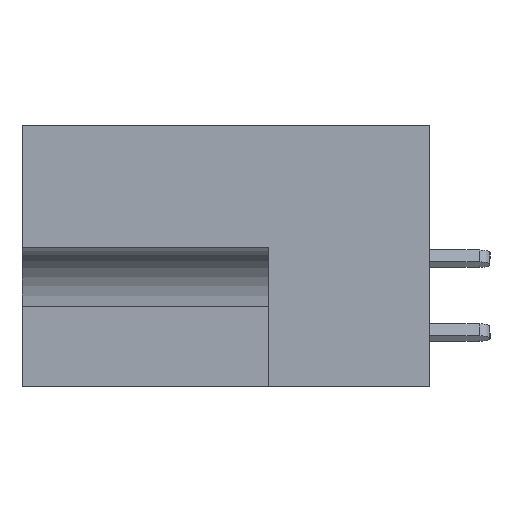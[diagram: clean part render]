
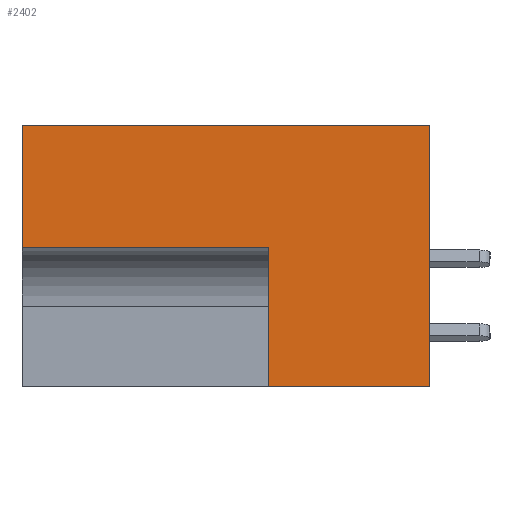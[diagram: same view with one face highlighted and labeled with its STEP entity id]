
A CAD part, left-side view. The second image highlights one B-rep face of the part: STEP entity #2402.
In plain terms, the highlighted planar face has unit normal (-1, 0, 0).
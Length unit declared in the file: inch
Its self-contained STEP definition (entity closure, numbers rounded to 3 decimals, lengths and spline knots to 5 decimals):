
#487 = VECTOR ( 'NONE', #11750, 39.37008 ) ;
#609 = EDGE_CURVE ( 'NONE', #8759, #22323, #5582, .T. ) ;
#642 = EDGE_CURVE ( 'NONE', #14120, #22938, #22885, .T. ) ;
#1224 = CARTESIAN_POINT ( 'NONE',  ( 0., 0.828, -0.248 ) ) ;
#1711 = EDGE_CURVE ( 'NONE', #22323, #21578, #14410, .T. ) ;
#2013 = CARTESIAN_POINT ( 'NONE',  ( 0., 0.453, -0.531 ) ) ;
#2112 = CARTESIAN_POINT ( 'NONE',  ( 0., 0.828, 0. ) ) ;
#2235 = CARTESIAN_POINT ( 'NONE',  ( 0., 0.328, -0.531 ) ) ;
#2402 = ADVANCED_FACE ( 'NONE', ( #11126 ), #15970, .F. ) ;
#2690 = EDGE_CURVE ( 'NONE', #22938, #19442, #9330, .T. ) ;
#3040 = VECTOR ( 'NONE', #19866, 39.37008 ) ;
#3917 = DIRECTION ( 'NONE',  ( 0., -1., 0. ) ) ;
#4312 = DIRECTION ( 'NONE',  ( 1., 0., 0. ) ) ;
#5582 = LINE ( 'NONE', #17254, #487 ) ;
#5792 = DIRECTION ( 'NONE',  ( 0., 0., 1. ) ) ;
#6482 = CARTESIAN_POINT ( 'NONE',  ( 0., 0.453, 0. ) ) ;
#7035 = ORIENTED_EDGE ( 'NONE', *, *, #1711, .F. ) ;
#7342 = EDGE_CURVE ( 'NONE', #14120, #8759, #15194, .T. ) ;
#7466 = ORIENTED_EDGE ( 'NONE', *, *, #609, .F. ) ;
#8346 = DIRECTION ( 'NONE',  ( 0., 0., 1. ) ) ;
#8411 = LINE ( 'NONE', #12101, #3040 ) ;
#8487 = VECTOR ( 'NONE', #10523, 39.37008 ) ;
#8759 = VERTEX_POINT ( 'NONE', #23006 ) ;
#9330 = LINE ( 'NONE', #20868, #13186 ) ;
#9802 = CARTESIAN_POINT ( 'NONE',  ( 0., 0.828, 0. ) ) ;
#10523 = DIRECTION ( 'NONE',  ( 0., 0., 1. ) ) ;
#10545 = EDGE_LOOP ( 'NONE', ( #7035, #7466, #19404, #20044, #15841, #23078 ) ) ;
#11126 = FACE_OUTER_BOUND ( 'NONE', #10545, .T. ) ;
#11750 = DIRECTION ( 'NONE',  ( 0., 1., 0. ) ) ;
#12101 = CARTESIAN_POINT ( 'NONE',  ( 0., 0.453, 0. ) ) ;
#12620 = CARTESIAN_POINT ( 'NONE',  ( 0., 0., 0. ) ) ;
#12725 = VECTOR ( 'NONE', #3917, 39.37008 ) ;
#13186 = VECTOR ( 'NONE', #5792, 39.37008 ) ;
#14005 = CARTESIAN_POINT ( 'NONE',  ( 0., 0.328, -0.531 ) ) ;
#14120 = VERTEX_POINT ( 'NONE', #2235 ) ;
#14410 = LINE ( 'NONE', #9802, #8487 ) ;
#15194 = LINE ( 'NONE', #14005, #15226 ) ;
#15226 = VECTOR ( 'NONE', #8346, 39.37008 ) ;
#15841 = ORIENTED_EDGE ( 'NONE', *, *, #2690, .T. ) ;
#15970 = PLANE ( 'NONE',  #17957 ) ;
#17254 = CARTESIAN_POINT ( 'NONE',  ( 0., 0.328, -0.248 ) ) ;
#17957 = AXIS2_PLACEMENT_3D ( 'NONE', #6482, #4312, #23334 ) ;
#19404 = ORIENTED_EDGE ( 'NONE', *, *, #7342, .F. ) ;
#19442 = VERTEX_POINT ( 'NONE', #12620 ) ;
#19866 = DIRECTION ( 'NONE',  ( 0., -1., 0. ) ) ;
#19978 = EDGE_CURVE ( 'NONE', #21578, #19442, #8411, .T. ) ;
#20044 = ORIENTED_EDGE ( 'NONE', *, *, #642, .T. ) ;
#20360 = CARTESIAN_POINT ( 'NONE',  ( 0., 0., -0.531 ) ) ;
#20868 = CARTESIAN_POINT ( 'NONE',  ( 0., 0., 0. ) ) ;
#21578 = VERTEX_POINT ( 'NONE', #2112 ) ;
#22323 = VERTEX_POINT ( 'NONE', #1224 ) ;
#22885 = LINE ( 'NONE', #2013, #12725 ) ;
#22938 = VERTEX_POINT ( 'NONE', #20360 ) ;
#23006 = CARTESIAN_POINT ( 'NONE',  ( 0., 0.328, -0.248 ) ) ;
#23078 = ORIENTED_EDGE ( 'NONE', *, *, #19978, .F. ) ;
#23334 = DIRECTION ( 'NONE',  ( 0., 0., -1. ) ) ;
